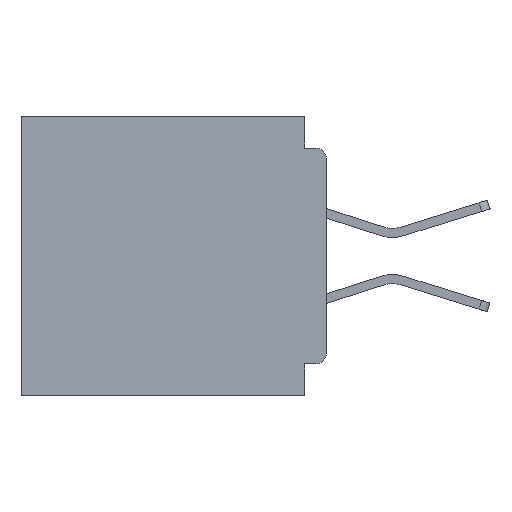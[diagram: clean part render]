
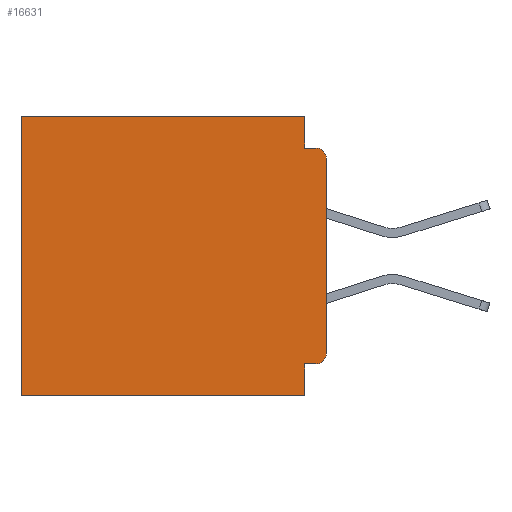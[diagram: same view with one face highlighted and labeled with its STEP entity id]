
A CAD part, left-side view. The second image highlights one B-rep face of the part: STEP entity #16631.
In plain terms, the highlighted planar face has unit normal (-1, 0, 0).
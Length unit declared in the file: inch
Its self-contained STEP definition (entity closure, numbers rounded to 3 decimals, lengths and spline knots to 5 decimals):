
#97 = ORIENTED_EDGE ( 'NONE', *, *, #10086, .T. ) ;
#286 = CARTESIAN_POINT ( 'NONE',  ( 0.3, 0.015, -0.34 ) ) ;
#2277 = AXIS2_PLACEMENT_3D ( 'NONE', #8578, #37954, #15951 ) ;
#2839 = ORIENTED_EDGE ( 'NONE', *, *, #39258, .T. ) ;
#3016 = CARTESIAN_POINT ( 'NONE',  ( 0.3, 0.437, -0.4 ) ) ;
#3017 = EDGE_CURVE ( 'NONE', #17714, #8985, #3556, .T. ) ;
#3556 = CIRCLE ( 'NONE', #22478, 0.015 ) ;
#3976 = DIRECTION ( 'NONE',  ( 0., 0., -1. ) ) ;
#4367 = DIRECTION ( 'NONE',  ( 0., 1., 0. ) ) ;
#4443 = ORIENTED_EDGE ( 'NONE', *, *, #45698, .F. ) ;
#4498 = VERTEX_POINT ( 'NONE', #39917 ) ;
#5256 = VECTOR ( 'NONE', #37585, 39.37008 ) ;
#7058 = VECTOR ( 'NONE', #24060, 39.37008 ) ;
#8578 = CARTESIAN_POINT ( 'NONE',  ( 0.3, 0., -0.4 ) ) ;
#8669 = EDGE_CURVE ( 'NONE', #13807, #11879, #26583, .T. ) ;
#8985 = VERTEX_POINT ( 'NONE', #22067 ) ;
#10086 = EDGE_CURVE ( 'NONE', #20760, #19486, #18811, .T. ) ;
#10410 = CARTESIAN_POINT ( 'NONE',  ( 0.3, 0.015, -0.06 ) ) ;
#10968 = ORIENTED_EDGE ( 'NONE', *, *, #8669, .F. ) ;
#10995 = AXIS2_PLACEMENT_3D ( 'NONE', #286, #25946, #3976 ) ;
#11220 = CARTESIAN_POINT ( 'NONE',  ( 0.3, 0., -0.06 ) ) ;
#11879 = VERTEX_POINT ( 'NONE', #3016 ) ;
#12236 = VECTOR ( 'NONE', #18448, 39.37008 ) ;
#13031 = ORIENTED_EDGE ( 'NONE', *, *, #23705, .F. ) ;
#13200 = DIRECTION ( 'NONE',  ( 0., 1., 0. ) ) ;
#13807 = VERTEX_POINT ( 'NONE', #19471 ) ;
#14826 = CARTESIAN_POINT ( 'NONE',  ( 0.3, 0., -0.34 ) ) ;
#15328 = VECTOR ( 'NONE', #19982, 39.37008 ) ;
#15696 = CARTESIAN_POINT ( 'NONE',  ( 0.3, 0.031, -0.4 ) ) ;
#15951 = DIRECTION ( 'NONE',  ( 0., 0., -1. ) ) ;
#16569 = VECTOR ( 'NONE', #29646, 39.37008 ) ;
#16631 = ADVANCED_FACE ( 'NONE', ( #24872 ), #26856, .F. ) ;
#16958 = ORIENTED_EDGE ( 'NONE', *, *, #29190, .F. ) ;
#17714 = VERTEX_POINT ( 'NONE', #11220 ) ;
#18298 = CARTESIAN_POINT ( 'NONE',  ( 0.3, 0., -0.4 ) ) ;
#18448 = DIRECTION ( 'NONE',  ( 0., 0., -1. ) ) ;
#18549 = CARTESIAN_POINT ( 'NONE',  ( 0.3, 0.437, -0.4 ) ) ;
#18811 = CIRCLE ( 'NONE', #10995, 0.015 ) ;
#19471 = CARTESIAN_POINT ( 'NONE',  ( 0.3, 0.031, -0.4 ) ) ;
#19486 = VERTEX_POINT ( 'NONE', #14826 ) ;
#19609 = CARTESIAN_POINT ( 'NONE',  ( 0.3, 0.031, -0.355 ) ) ;
#19698 = ORIENTED_EDGE ( 'NONE', *, *, #30705, .T. ) ;
#19982 = DIRECTION ( 'NONE',  ( 0., -1., 0. ) ) ;
#20328 = EDGE_CURVE ( 'NONE', #29056, #13807, #27357, .T. ) ;
#20354 = CARTESIAN_POINT ( 'NONE',  ( 0.3, 0., -0.4 ) ) ;
#20760 = VERTEX_POINT ( 'NONE', #32665 ) ;
#21957 = LINE ( 'NONE', #18298, #12236 ) ;
#22067 = CARTESIAN_POINT ( 'NONE',  ( 0.3, 0.015, -0.045 ) ) ;
#22444 = VERTEX_POINT ( 'NONE', #30844 ) ;
#22478 = AXIS2_PLACEMENT_3D ( 'NONE', #10410, #36371, #33646 ) ;
#22881 = VERTEX_POINT ( 'NONE', #40916 ) ;
#23331 = ORIENTED_EDGE ( 'NONE', *, *, #45861, .F. ) ;
#23705 = EDGE_CURVE ( 'NONE', #22444, #8985, #43419, .T. ) ;
#24060 = DIRECTION ( 'NONE',  ( 0., 1., 0. ) ) ;
#24872 = FACE_OUTER_BOUND ( 'NONE', #34739, .T. ) ;
#25946 = DIRECTION ( 'NONE',  ( -1., 0., 0. ) ) ;
#26353 = CARTESIAN_POINT ( 'NONE',  ( 0.3, 0., 0. ) ) ;
#26583 = LINE ( 'NONE', #20354, #7058 ) ;
#26856 = PLANE ( 'NONE',  #2277 ) ;
#27357 = LINE ( 'NONE', #15696, #34863 ) ;
#29056 = VERTEX_POINT ( 'NONE', #19609 ) ;
#29190 = EDGE_CURVE ( 'NONE', #20760, #29056, #31703, .T. ) ;
#29646 = DIRECTION ( 'NONE',  ( 0., 0., -1. ) ) ;
#30186 = CARTESIAN_POINT ( 'NONE',  ( 0.3, 0.031, 0. ) ) ;
#30705 = EDGE_CURVE ( 'NONE', #22881, #11879, #36127, .T. ) ;
#30844 = CARTESIAN_POINT ( 'NONE',  ( 0.3, 0.031, -0.045 ) ) ;
#31703 = LINE ( 'NONE', #35189, #41478 ) ;
#32078 = LINE ( 'NONE', #26353, #41860 ) ;
#32665 = CARTESIAN_POINT ( 'NONE',  ( 0.3, 0.015, -0.355 ) ) ;
#33646 = DIRECTION ( 'NONE',  ( 0., 0., -1. ) ) ;
#34739 = EDGE_LOOP ( 'NONE', ( #4443, #41464, #13031, #23331, #2839, #19698, #10968, #46439, #16958, #97 ) ) ;
#34863 = VECTOR ( 'NONE', #37723, 39.37008 ) ;
#35189 = CARTESIAN_POINT ( 'NONE',  ( 0.3, 0., -0.355 ) ) ;
#36127 = LINE ( 'NONE', #18549, #16569 ) ;
#36371 = DIRECTION ( 'NONE',  ( -1., 0., 0. ) ) ;
#37585 = DIRECTION ( 'NONE',  ( 0., 0., -1. ) ) ;
#37723 = DIRECTION ( 'NONE',  ( 0., 0., -1. ) ) ;
#37954 = DIRECTION ( 'NONE',  ( 1., 0., 0. ) ) ;
#39258 = EDGE_CURVE ( 'NONE', #4498, #22881, #32078, .T. ) ;
#39917 = CARTESIAN_POINT ( 'NONE',  ( 0.3, 0.031, 0. ) ) ;
#40916 = CARTESIAN_POINT ( 'NONE',  ( 0.3, 0.437, 0. ) ) ;
#41464 = ORIENTED_EDGE ( 'NONE', *, *, #3017, .T. ) ;
#41478 = VECTOR ( 'NONE', #13200, 39.37008 ) ;
#41860 = VECTOR ( 'NONE', #4367, 39.37008 ) ;
#41958 = CARTESIAN_POINT ( 'NONE',  ( 0.3, 0., -0.045 ) ) ;
#43419 = LINE ( 'NONE', #41958, #15328 ) ;
#44290 = LINE ( 'NONE', #30186, #5256 ) ;
#45698 = EDGE_CURVE ( 'NONE', #17714, #19486, #21957, .T. ) ;
#45861 = EDGE_CURVE ( 'NONE', #4498, #22444, #44290, .T. ) ;
#46439 = ORIENTED_EDGE ( 'NONE', *, *, #20328, .F. ) ;
